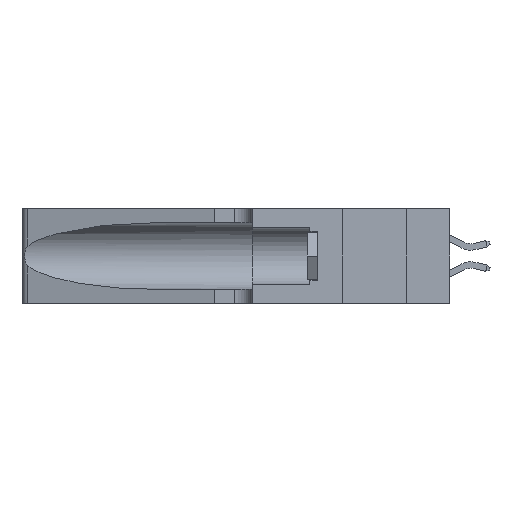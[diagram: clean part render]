
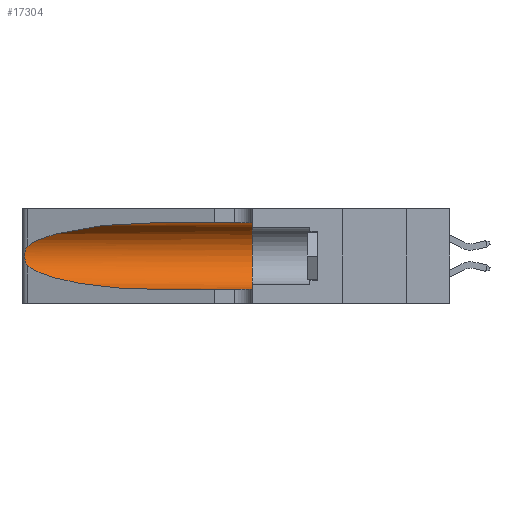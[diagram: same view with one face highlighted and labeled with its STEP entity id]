
A CAD part, left-side view. The second image highlights one B-rep face of the part: STEP entity #17304.
In plain terms, the highlighted cylindrical face has radius 3.308 mm (diameter 6.617 mm), a partial arc.
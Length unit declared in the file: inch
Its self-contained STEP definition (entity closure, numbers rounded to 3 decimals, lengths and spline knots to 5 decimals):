
#257 =( BOUNDED_CURVE ( )  B_SPLINE_CURVE ( 3, ( #20152, #14521, #18255, #8959 ),
 .UNSPECIFIED., .F., .T. ) 
 B_SPLINE_CURVE_WITH_KNOTS ( ( 4, 4 ),
 ( 3.44316, 4.71239 ),
 .UNSPECIFIED. ) 
 CURVE ( )  GEOMETRIC_REPRESENTATION_ITEM ( )  RATIONAL_B_SPLINE_CURVE ( ( 1., 0.87, 0.87, 1. ) ) 
 REPRESENTATION_ITEM ( '' )  );
#514 = CARTESIAN_POINT ( 'NONE',  ( 0.25487, 1.22718, 0.14631 ) ) ;
#613 = ORIENTED_EDGE ( 'NONE', *, *, #10407, .T. ) ;
#979 = CARTESIAN_POINT ( 'NONE',  ( 0.1305, 0.72297, 0.31525 ) ) ;
#1073 = CYLINDRICAL_SURFACE ( 'NONE', #17242, 0.13025 ) ;
#1137 = CARTESIAN_POINT ( 'NONE',  ( 0.25555, 1.22994, 0.2215 ) ) ;
#1222 = CARTESIAN_POINT ( 'NONE',  ( 0.26017, 1.23833, 0.17102 ) ) ;
#1687 = FACE_OUTER_BOUND ( 'NONE', #14565, .T. ) ;
#3198 = CARTESIAN_POINT ( 'NONE',  ( 0.25789, 1.23486, 0.15765 ) ) ;
#3537 = CARTESIAN_POINT ( 'NONE',  ( 0.1305, 0.35, 0.31525 ) ) ;
#3613 = VERTEX_POINT ( 'NONE', #979 ) ;
#4460 = ORIENTED_EDGE ( 'NONE', *, *, #7567, .T. ) ;
#4670 = DIRECTION ( 'NONE',  ( 0., -1., 0. ) ) ;
#4782 = VERTEX_POINT ( 'NONE', #8543 ) ;
#4934 = EDGE_CURVE ( 'NONE', #14377, #14854, #257, .T. ) ;
#5114 = CARTESIAN_POINT ( 'NONE',  ( 0.25555, 1.22993, 0.14849 ) ) ;
#5641 = DIRECTION ( 'NONE',  ( 0., -1., 0. ) ) ;
#5714 = CARTESIAN_POINT ( 'NONE',  ( 0.1305, 0.72297, 0.05475 ) ) ;
#5875 = DIRECTION ( 'NONE',  ( 0., -1., 0. ) ) ;
#6564 = DIRECTION ( 'NONE',  ( 0., 0., -1. ) ) ;
#7143 = CARTESIAN_POINT ( 'NONE',  ( 0.1305, 0.35, 0.185 ) ) ;
#7567 = EDGE_CURVE ( 'NONE', #3613, #4782, #20394, .T. ) ;
#8339 = CIRCLE ( 'NONE', #22167, 0.13025 ) ;
#8524 = CARTESIAN_POINT ( 'NONE',  ( 0.2373, 1.15595, 0.28018 ) ) ;
#8543 = CARTESIAN_POINT ( 'NONE',  ( 0.25487, 1.22718, 0.22369 ) ) ;
#8753 = CARTESIAN_POINT ( 'NONE',  ( 0.25487, 1.22718, 0.22369 ) ) ;
#8827 = CARTESIAN_POINT ( 'NONE',  ( 0.25787, 1.23484, 0.2124 ) ) ;
#8959 = CARTESIAN_POINT ( 'NONE',  ( 0.1305, 0.72297, 0.05475 ) ) ;
#9048 = DIRECTION ( 'NONE',  ( 0., 0., 1. ) ) ;
#9354 = EDGE_CURVE ( 'NONE', #3613, #18449, #14807, .T. ) ;
#9690 = ORIENTED_EDGE ( 'NONE', *, *, #14011, .T. ) ;
#10106 = ORIENTED_EDGE ( 'NONE', *, *, #20907, .F. ) ;
#10407 = EDGE_CURVE ( 'NONE', #14854, #14165, #24400, .T. ) ;
#10699 = CARTESIAN_POINT ( 'NONE',  ( 0.26018, 1.23835, 0.19895 ) ) ;
#11534 = CARTESIAN_POINT ( 'NONE',  ( 0.1305, 1.61858, 0.31525 ) ) ;
#11679 = B_SPLINE_CURVE_WITH_KNOTS ( 'NONE', 3,
 ( #8753, #1137, #20024, #8827, #21907, #10699, #23789, #12580, #1222, #14474, #3198, #16321, #5114, #18209 ),
 .UNSPECIFIED., .F., .F.,
 ( 4, 2, 2, 2, 2, 2, 4 ),
 ( 0., 0.00027, 0.00053, 0.00107, 0.0016, 0.00187, 0.00214 ),
 .UNSPECIFIED. ) ;
#12580 = CARTESIAN_POINT ( 'NONE',  ( 0.26075, 1.23896, 0.178 ) ) ;
#14011 = EDGE_CURVE ( 'NONE', #4782, #14377, #11679, .T. ) ;
#14095 = CARTESIAN_POINT ( 'NONE',  ( 0.1305, 0.72297, 0.31525 ) ) ;
#14165 = VERTEX_POINT ( 'NONE', #18774 ) ;
#14377 = VERTEX_POINT ( 'NONE', #514 ) ;
#14474 = CARTESIAN_POINT ( 'NONE',  ( 0.25856, 1.23593, 0.16098 ) ) ;
#14521 = CARTESIAN_POINT ( 'NONE',  ( 0.2373, 1.15595, 0.08982 ) ) ;
#14565 = EDGE_LOOP ( 'NONE', ( #4460, #9690, #20175, #613, #10106, #15022 ) ) ;
#14807 = LINE ( 'NONE', #11534, #19774 ) ;
#14854 = VERTEX_POINT ( 'NONE', #5714 ) ;
#15022 = ORIENTED_EDGE ( 'NONE', *, *, #9354, .F. ) ;
#15620 = VECTOR ( 'NONE', #5641, 39.37008 ) ;
#16321 = CARTESIAN_POINT ( 'NONE',  ( 0.25639, 1.23186, 0.15144 ) ) ;
#16870 = CARTESIAN_POINT ( 'NONE',  ( 0.1305, 1.61858, 0.05475 ) ) ;
#17242 = AXIS2_PLACEMENT_3D ( 'NONE', #17758, #4670, #6564 ) ;
#17304 = ADVANCED_FACE ( 'NONE', ( #1687 ), #1073, .F. ) ;
#17752 = CARTESIAN_POINT ( 'NONE',  ( 0.18966, 0.96281, 0.31525 ) ) ;
#17758 = CARTESIAN_POINT ( 'NONE',  ( 0.1305, 1.61858, 0.185 ) ) ;
#18209 = CARTESIAN_POINT ( 'NONE',  ( 0.25487, 1.22718, 0.14631 ) ) ;
#18255 = CARTESIAN_POINT ( 'NONE',  ( 0.18966, 0.96281, 0.05475 ) ) ;
#18449 = VERTEX_POINT ( 'NONE', #3537 ) ;
#18774 = CARTESIAN_POINT ( 'NONE',  ( 0.1305, 0.35, 0.05475 ) ) ;
#19774 = VECTOR ( 'NONE', #5875, 39.37008 ) ;
#20024 = CARTESIAN_POINT ( 'NONE',  ( 0.25639, 1.23184, 0.21858 ) ) ;
#20152 = CARTESIAN_POINT ( 'NONE',  ( 0.25487, 1.22718, 0.14631 ) ) ;
#20175 = ORIENTED_EDGE ( 'NONE', *, *, #4934, .T. ) ;
#20242 = DIRECTION ( 'NONE',  ( 0., 1., 0. ) ) ;
#20394 =( BOUNDED_CURVE ( )  B_SPLINE_CURVE ( 3, ( #14095, #17752, #8524, #21618 ),
 .UNSPECIFIED., .F., .T. ) 
 B_SPLINE_CURVE_WITH_KNOTS ( ( 4, 4 ),
 ( 1.5708, 2.84003 ),
 .UNSPECIFIED. ) 
 CURVE ( )  GEOMETRIC_REPRESENTATION_ITEM ( )  RATIONAL_B_SPLINE_CURVE ( ( 1., 0.87, 0.87, 1. ) ) 
 REPRESENTATION_ITEM ( '' )  );
#20907 = EDGE_CURVE ( 'NONE', #18449, #14165, #8339, .T. ) ;
#21618 = CARTESIAN_POINT ( 'NONE',  ( 0.25487, 1.22718, 0.22369 ) ) ;
#21907 = CARTESIAN_POINT ( 'NONE',  ( 0.25854, 1.2359, 0.20912 ) ) ;
#22167 = AXIS2_PLACEMENT_3D ( 'NONE', #7143, #20242, #9048 ) ;
#23789 = CARTESIAN_POINT ( 'NONE',  ( 0.26075, 1.23896, 0.19203 ) ) ;
#24400 = LINE ( 'NONE', #16870, #15620 ) ;
